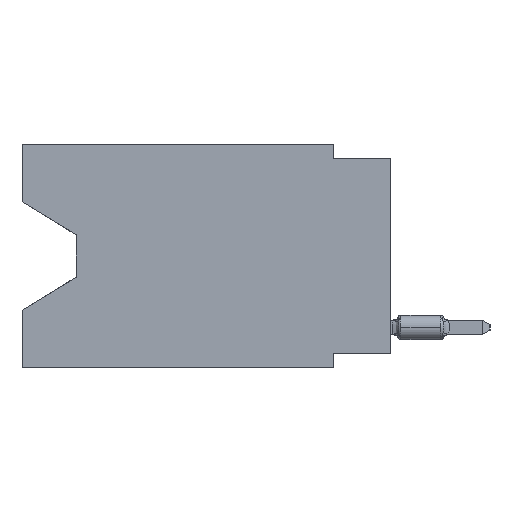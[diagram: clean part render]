
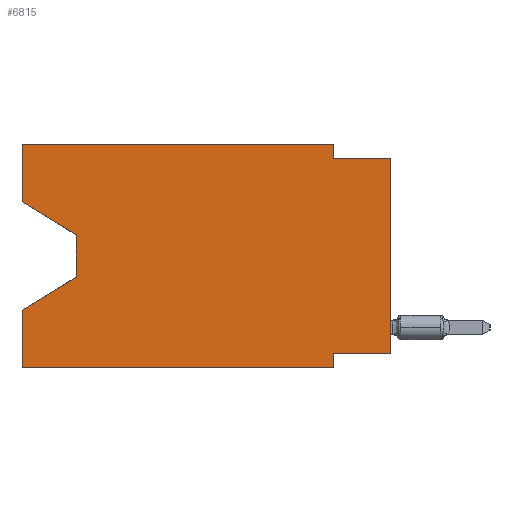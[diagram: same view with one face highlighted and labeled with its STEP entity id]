
A CAD part, left-side view. The second image highlights one B-rep face of the part: STEP entity #6815.
In plain terms, the highlighted planar face has unit normal (-1, 0, 0).
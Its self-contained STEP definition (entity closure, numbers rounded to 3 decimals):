
#106 = LINE ( 'NONE', #4887, #15293 ) ;
#420 = EDGE_LOOP ( 'NONE', ( #6290, #8538, #1973, #14332, #7964, #3803, #4455, #12886, #8585, #1247, #1958, #15717 ) ) ;
#764 = CARTESIAN_POINT ( 'NONE',  ( 0., 16.383, 0. ) ) ;
#1247 = ORIENTED_EDGE ( 'NONE', *, *, #1779, .F. ) ;
#1268 = VERTEX_POINT ( 'NONE', #12098 ) ;
#1313 = VECTOR ( 'NONE', #15403, 1000. ) ;
#1563 = VERTEX_POINT ( 'NONE', #13347 ) ;
#1693 = DIRECTION ( 'NONE',  ( 0., 0., 1. ) ) ;
#1764 = VECTOR ( 'NONE', #14710, 1000. ) ;
#1779 = EDGE_CURVE ( 'NONE', #20636, #7126, #18965, .T. ) ;
#1836 = DIRECTION ( 'NONE',  ( 0., -0.855, -0.519 ) ) ;
#1958 = ORIENTED_EDGE ( 'NONE', *, *, #18790, .F. ) ;
#1973 = ORIENTED_EDGE ( 'NONE', *, *, #18581, .T. ) ;
#2271 = DIRECTION ( 'NONE',  ( 0., 0., -1. ) ) ;
#2372 = CARTESIAN_POINT ( 'NONE',  ( 0., 16.383, 0. ) ) ;
#2590 = VERTEX_POINT ( 'NONE', #13722 ) ;
#3461 = CARTESIAN_POINT ( 'NONE',  ( 0., 16.383, 0. ) ) ;
#3653 = PLANE ( 'NONE',  #7083 ) ;
#3666 = DIRECTION ( 'NONE',  ( 0., -1., 0. ) ) ;
#3712 = VERTEX_POINT ( 'NONE', #20722 ) ;
#3803 = ORIENTED_EDGE ( 'NONE', *, *, #10554, .F. ) ;
#4315 = CARTESIAN_POINT ( 'NONE',  ( 0., 2.54, -9.906 ) ) ;
#4346 = EDGE_CURVE ( 'NONE', #15836, #1563, #14862, .T. ) ;
#4455 = ORIENTED_EDGE ( 'NONE', *, *, #13683, .F. ) ;
#4887 = CARTESIAN_POINT ( 'NONE',  ( 0., 0., 0. ) ) ;
#5247 = CARTESIAN_POINT ( 'NONE',  ( 0., 16.383, 0. ) ) ;
#5338 = LINE ( 'NONE', #16294, #1764 ) ;
#5411 = CARTESIAN_POINT ( 'NONE',  ( 0., 0., -0.635 ) ) ;
#5564 = DIRECTION ( 'NONE',  ( 1., 0., 0. ) ) ;
#6290 = ORIENTED_EDGE ( 'NONE', *, *, #14297, .T. ) ;
#6805 = LINE ( 'NONE', #16502, #13109 ) ;
#6815 = ADVANCED_FACE ( 'NONE', ( #18105 ), #3653, .F. ) ;
#7083 = AXIS2_PLACEMENT_3D ( 'NONE', #2372, #5564, #2271 ) ;
#7126 = VERTEX_POINT ( 'NONE', #14806 ) ;
#7158 = VECTOR ( 'NONE', #18295, 1000. ) ;
#7272 = DIRECTION ( 'NONE',  ( 0., 0., -1. ) ) ;
#7350 = EDGE_CURVE ( 'NONE', #11943, #20155, #16999, .T. ) ;
#7964 = ORIENTED_EDGE ( 'NONE', *, *, #7350, .T. ) ;
#8150 = VERTEX_POINT ( 'NONE', #12178 ) ;
#8407 = VERTEX_POINT ( 'NONE', #9811 ) ;
#8538 = ORIENTED_EDGE ( 'NONE', *, *, #20993, .T. ) ;
#8585 = ORIENTED_EDGE ( 'NONE', *, *, #17857, .F. ) ;
#9709 = DIRECTION ( 'NONE',  ( 0., 0., -1. ) ) ;
#9811 = CARTESIAN_POINT ( 'NONE',  ( 0., 13.97, -5.893 ) ) ;
#10192 = CARTESIAN_POINT ( 'NONE',  ( 0., 16.383, -9.906 ) ) ;
#10202 = VECTOR ( 'NONE', #10253, 1000. ) ;
#10253 = DIRECTION ( 'NONE',  ( 0., 0., 1. ) ) ;
#10376 = VECTOR ( 'NONE', #20997, 1000. ) ;
#10554 = EDGE_CURVE ( 'NONE', #2590, #20155, #5338, .T. ) ;
#11825 = CARTESIAN_POINT ( 'NONE',  ( 0., 0., -9.271 ) ) ;
#11943 = VERTEX_POINT ( 'NONE', #10192 ) ;
#12073 = VECTOR ( 'NONE', #9709, 1000. ) ;
#12098 = CARTESIAN_POINT ( 'NONE',  ( 0., 0., -9.271 ) ) ;
#12178 = CARTESIAN_POINT ( 'NONE',  ( 0., 16.383, -7.36 ) ) ;
#12377 = CARTESIAN_POINT ( 'NONE',  ( 0., 13.97, -4.013 ) ) ;
#12419 = CARTESIAN_POINT ( 'NONE',  ( 0., 16.383, -9.906 ) ) ;
#12791 = EDGE_CURVE ( 'NONE', #11943, #8150, #13550, .T. ) ;
#12886 = ORIENTED_EDGE ( 'NONE', *, *, #13124, .T. ) ;
#13013 = CARTESIAN_POINT ( 'NONE',  ( 0., 16.383, -2.546 ) ) ;
#13109 = VECTOR ( 'NONE', #18198, 1000. ) ;
#13124 = EDGE_CURVE ( 'NONE', #1268, #18370, #106, .T. ) ;
#13248 = VECTOR ( 'NONE', #7272, 1000. ) ;
#13343 = LINE ( 'NONE', #5247, #14459 ) ;
#13347 = CARTESIAN_POINT ( 'NONE',  ( 0., 16.383, 0. ) ) ;
#13398 = VECTOR ( 'NONE', #16331, 1000. ) ;
#13550 = LINE ( 'NONE', #764, #10202 ) ;
#13683 = EDGE_CURVE ( 'NONE', #1268, #2590, #19907, .T. ) ;
#13722 = CARTESIAN_POINT ( 'NONE',  ( 0., 2.54, -9.271 ) ) ;
#13779 = CARTESIAN_POINT ( 'NONE',  ( 0., 2.54, 0. ) ) ;
#14297 = EDGE_CURVE ( 'NONE', #15836, #3712, #19826, .T. ) ;
#14332 = ORIENTED_EDGE ( 'NONE', *, *, #12791, .F. ) ;
#14459 = VECTOR ( 'NONE', #3666, 1000. ) ;
#14496 = CARTESIAN_POINT ( 'NONE',  ( 0., 2.54, 0. ) ) ;
#14623 = LINE ( 'NONE', #18114, #10376 ) ;
#14661 = VECTOR ( 'NONE', #1836, 1000. ) ;
#14710 = DIRECTION ( 'NONE',  ( 0., 0., -1. ) ) ;
#14806 = CARTESIAN_POINT ( 'NONE',  ( 0., 2.54, -0.635 ) ) ;
#14862 = LINE ( 'NONE', #3461, #13398 ) ;
#15293 = VECTOR ( 'NONE', #1693, 1000. ) ;
#15403 = DIRECTION ( 'NONE',  ( 0., -1., 0. ) ) ;
#15717 = ORIENTED_EDGE ( 'NONE', *, *, #4346, .F. ) ;
#15836 = VERTEX_POINT ( 'NONE', #16100 ) ;
#16100 = CARTESIAN_POINT ( 'NONE',  ( 0., 16.383, -2.546 ) ) ;
#16294 = CARTESIAN_POINT ( 'NONE',  ( 0., 2.54, -9.906 ) ) ;
#16331 = DIRECTION ( 'NONE',  ( 0., 0., 1. ) ) ;
#16502 = CARTESIAN_POINT ( 'NONE',  ( 0., 0., -0.635 ) ) ;
#16999 = LINE ( 'NONE', #12419, #1313 ) ;
#17061 = LINE ( 'NONE', #12377, #13248 ) ;
#17857 = EDGE_CURVE ( 'NONE', #7126, #18370, #6805, .T. ) ;
#18105 = FACE_OUTER_BOUND ( 'NONE', #420, .T. ) ;
#18114 = CARTESIAN_POINT ( 'NONE',  ( 0., 13.97, -5.893 ) ) ;
#18198 = DIRECTION ( 'NONE',  ( 0., -1., 0. ) ) ;
#18295 = DIRECTION ( 'NONE',  ( 0., 1., 0. ) ) ;
#18370 = VERTEX_POINT ( 'NONE', #5411 ) ;
#18581 = EDGE_CURVE ( 'NONE', #8407, #8150, #14623, .T. ) ;
#18790 = EDGE_CURVE ( 'NONE', #1563, #20636, #13343, .T. ) ;
#18965 = LINE ( 'NONE', #14496, #12073 ) ;
#19826 = LINE ( 'NONE', #13013, #14661 ) ;
#19907 = LINE ( 'NONE', #11825, #7158 ) ;
#20155 = VERTEX_POINT ( 'NONE', #4315 ) ;
#20636 = VERTEX_POINT ( 'NONE', #13779 ) ;
#20722 = CARTESIAN_POINT ( 'NONE',  ( 0., 13.97, -4.013 ) ) ;
#20993 = EDGE_CURVE ( 'NONE', #3712, #8407, #17061, .T. ) ;
#20997 = DIRECTION ( 'NONE',  ( 0., 0.855, -0.519 ) ) ;
